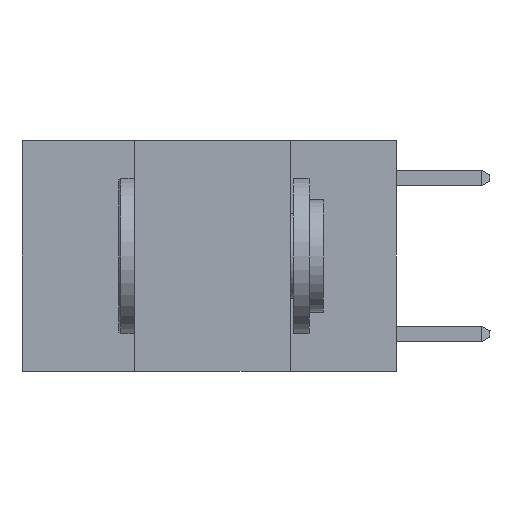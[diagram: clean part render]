
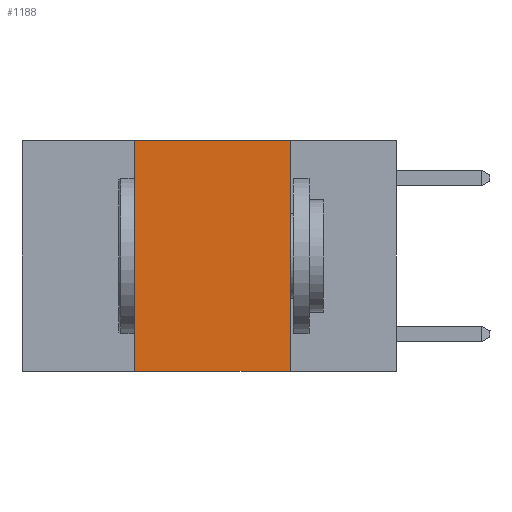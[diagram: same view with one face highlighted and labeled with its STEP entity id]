
A CAD part, left-side view. The second image highlights one B-rep face of the part: STEP entity #1188.
In plain terms, the highlighted planar face has unit normal (-1, 0, 0).
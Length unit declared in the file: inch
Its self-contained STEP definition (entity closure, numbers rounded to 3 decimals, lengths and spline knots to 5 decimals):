
#586 = VECTOR ( 'NONE', #676, 39.37008 ) ;
#676 = DIRECTION ( 'NONE',  ( 0., -1., 0. ) ) ;
#901 = VERTEX_POINT ( 'NONE', #16884 ) ;
#1188 = ADVANCED_FACE ( 'NONE', ( #9549 ), #13921, .F. ) ;
#4471 = LINE ( 'NONE', #11593, #13627 ) ;
#5739 = VERTEX_POINT ( 'NONE', #16243 ) ;
#6664 = LINE ( 'NONE', #9620, #13847 ) ;
#6763 = EDGE_CURVE ( 'NONE', #8756, #5739, #4471, .T. ) ;
#7125 = ORIENTED_EDGE ( 'NONE', *, *, #9053, .F. ) ;
#7208 = CARTESIAN_POINT ( 'NONE',  ( 0., 0.17, 0. ) ) ;
#7243 = ORIENTED_EDGE ( 'NONE', *, *, #14842, .T. ) ;
#8210 = EDGE_CURVE ( 'NONE', #11115, #901, #10396, .T. ) ;
#8756 = VERTEX_POINT ( 'NONE', #11752 ) ;
#9053 = EDGE_CURVE ( 'NONE', #5739, #11115, #13381, .T. ) ;
#9130 = AXIS2_PLACEMENT_3D ( 'NONE', #12311, #16595, #12412 ) ;
#9233 = ORIENTED_EDGE ( 'NONE', *, *, #8210, .F. ) ;
#9549 = FACE_OUTER_BOUND ( 'NONE', #10365, .T. ) ;
#9620 = CARTESIAN_POINT ( 'NONE',  ( 0., 0.6, -0.37 ) ) ;
#10365 = EDGE_LOOP ( 'NONE', ( #9233, #7125, #16868, #7243 ) ) ;
#10396 = LINE ( 'NONE', #14695, #15275 ) ;
#11115 = VERTEX_POINT ( 'NONE', #7208 ) ;
#11593 = CARTESIAN_POINT ( 'NONE',  ( 0., 0.42, 0. ) ) ;
#11752 = CARTESIAN_POINT ( 'NONE',  ( 0., 0.42, -0.37 ) ) ;
#12111 = DIRECTION ( 'NONE',  ( 0., -1., 0. ) ) ;
#12311 = CARTESIAN_POINT ( 'NONE',  ( 0., 0.6, 0. ) ) ;
#12412 = DIRECTION ( 'NONE',  ( 0., 0., -1. ) ) ;
#13381 = LINE ( 'NONE', #13574, #586 ) ;
#13574 = CARTESIAN_POINT ( 'NONE',  ( 0., 0.6, 0. ) ) ;
#13627 = VECTOR ( 'NONE', #17251, 39.37008 ) ;
#13847 = VECTOR ( 'NONE', #12111, 39.37008 ) ;
#13921 = PLANE ( 'NONE',  #9130 ) ;
#14695 = CARTESIAN_POINT ( 'NONE',  ( 0., 0.17, 0. ) ) ;
#14842 = EDGE_CURVE ( 'NONE', #8756, #901, #6664, .T. ) ;
#14885 = DIRECTION ( 'NONE',  ( 0., 0., -1. ) ) ;
#15275 = VECTOR ( 'NONE', #14885, 39.37008 ) ;
#16243 = CARTESIAN_POINT ( 'NONE',  ( 0., 0.42, 0. ) ) ;
#16595 = DIRECTION ( 'NONE',  ( 1., 0., 0. ) ) ;
#16868 = ORIENTED_EDGE ( 'NONE', *, *, #6763, .F. ) ;
#16884 = CARTESIAN_POINT ( 'NONE',  ( 0., 0.17, -0.37 ) ) ;
#17251 = DIRECTION ( 'NONE',  ( 0., 0., 1. ) ) ;
